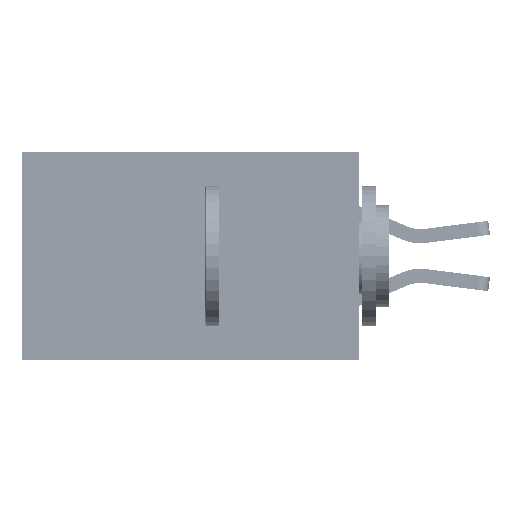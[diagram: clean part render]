
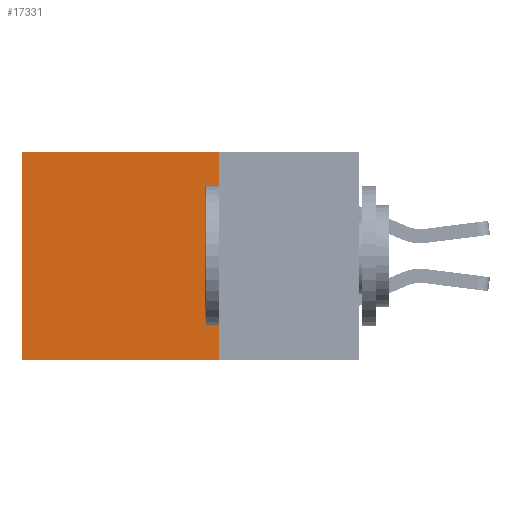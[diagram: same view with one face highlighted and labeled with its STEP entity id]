
A CAD part, left-side view. The second image highlights one B-rep face of the part: STEP entity #17331.
In plain terms, the highlighted planar face has unit normal (-1, 0, 0).
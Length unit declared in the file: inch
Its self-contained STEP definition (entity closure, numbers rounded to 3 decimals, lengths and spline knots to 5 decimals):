
#269 = EDGE_LOOP ( 'NONE', ( #6820, #31333, #39032, #28738 ) ) ;
#753 = DIRECTION ( 'NONE',  ( 0., 0., -1. ) ) ;
#1898 = LINE ( 'NONE', #4694, #31276 ) ;
#2774 = VERTEX_POINT ( 'NONE', #4906 ) ;
#4694 = CARTESIAN_POINT ( 'NONE',  ( 0.2875, 0.25, -0.37 ) ) ;
#4906 = CARTESIAN_POINT ( 'NONE',  ( 0.2875, 0.6, 0. ) ) ;
#4963 = CARTESIAN_POINT ( 'NONE',  ( 0.2875, 0.25, -0.37 ) ) ;
#4999 = CARTESIAN_POINT ( 'NONE',  ( 0.2875, 0.6, -0.37 ) ) ;
#5610 = VECTOR ( 'NONE', #753, 39.37008 ) ;
#6138 = VECTOR ( 'NONE', #35059, 39.37008 ) ;
#6344 = VECTOR ( 'NONE', #38770, 39.37008 ) ;
#6820 = ORIENTED_EDGE ( 'NONE', *, *, #19086, .T. ) ;
#7834 = AXIS2_PLACEMENT_3D ( 'NONE', #31811, #12815, #22455 ) ;
#8884 = FACE_OUTER_BOUND ( 'NONE', #269, .T. ) ;
#9270 = CARTESIAN_POINT ( 'NONE',  ( 0.2875, 0.25, 0. ) ) ;
#10217 = EDGE_CURVE ( 'NONE', #37857, #37612, #25229, .T. ) ;
#12815 = DIRECTION ( 'NONE',  ( 1., 0., 0. ) ) ;
#13578 = CARTESIAN_POINT ( 'NONE',  ( 0.2875, 0.6, 0. ) ) ;
#15641 = LINE ( 'NONE', #29081, #6344 ) ;
#15982 = CARTESIAN_POINT ( 'NONE',  ( 0.2875, 0.25, 0. ) ) ;
#17331 = ADVANCED_FACE ( 'NONE', ( #8884 ), #19037, .F. ) ;
#19037 = PLANE ( 'NONE',  #7834 ) ;
#19086 = EDGE_CURVE ( 'NONE', #2774, #35670, #25214, .T. ) ;
#21383 = EDGE_CURVE ( 'NONE', #37857, #2774, #15641, .T. ) ;
#22455 = DIRECTION ( 'NONE',  ( 0., 0., -1. ) ) ;
#25214 = LINE ( 'NONE', #13578, #5610 ) ;
#25229 = LINE ( 'NONE', #15982, #6138 ) ;
#26442 = DIRECTION ( 'NONE',  ( 0., 1., 0. ) ) ;
#28738 = ORIENTED_EDGE ( 'NONE', *, *, #21383, .T. ) ;
#29081 = CARTESIAN_POINT ( 'NONE',  ( 0.2875, 0.25, 0. ) ) ;
#31276 = VECTOR ( 'NONE', #26442, 39.37008 ) ;
#31333 = ORIENTED_EDGE ( 'NONE', *, *, #34094, .F. ) ;
#31811 = CARTESIAN_POINT ( 'NONE',  ( 0.2875, 0.25, 0. ) ) ;
#34094 = EDGE_CURVE ( 'NONE', #37612, #35670, #1898, .T. ) ;
#35059 = DIRECTION ( 'NONE',  ( 0., 0., -1. ) ) ;
#35670 = VERTEX_POINT ( 'NONE', #4999 ) ;
#37612 = VERTEX_POINT ( 'NONE', #4963 ) ;
#37857 = VERTEX_POINT ( 'NONE', #9270 ) ;
#38770 = DIRECTION ( 'NONE',  ( 0., 1., 0. ) ) ;
#39032 = ORIENTED_EDGE ( 'NONE', *, *, #10217, .F. ) ;
